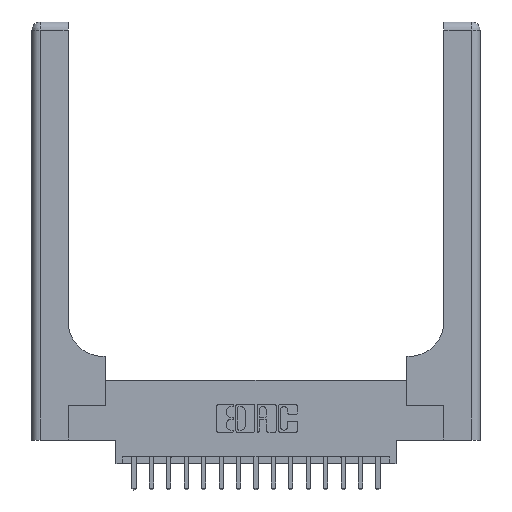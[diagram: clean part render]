
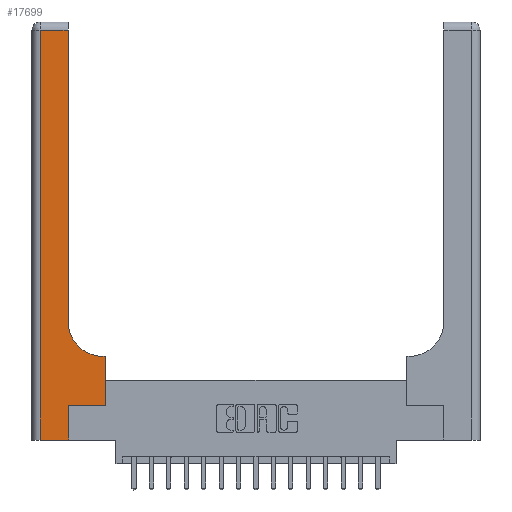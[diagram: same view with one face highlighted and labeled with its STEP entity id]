
A CAD part, top view. The second image highlights one B-rep face of the part: STEP entity #17699.
In plain terms, the highlighted planar face has unit normal (0, 0, 1).
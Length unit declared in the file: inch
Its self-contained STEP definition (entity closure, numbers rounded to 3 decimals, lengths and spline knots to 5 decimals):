
#5 = VERTEX_POINT ( 'NONE', #7284 ) ;
#361 = ORIENTED_EDGE ( 'NONE', *, *, #1503, .T. ) ;
#871 = CARTESIAN_POINT ( 'NONE',  ( 0.265, 0.25, 0.37 ) ) ;
#1188 = ORIENTED_EDGE ( 'NONE', *, *, #7287, .T. ) ;
#1314 = LINE ( 'NONE', #4271, #15556 ) ;
#1371 = CARTESIAN_POINT ( 'NONE',  ( 0.51, 0.6, 0.37 ) ) ;
#1503 = EDGE_CURVE ( 'NONE', #2085, #4782, #2754, .T. ) ;
#1678 = VECTOR ( 'NONE', #9289, 39.37008 ) ;
#1714 = EDGE_CURVE ( 'NONE', #8407, #12423, #7876, .T. ) ;
#2085 = VERTEX_POINT ( 'NONE', #15450 ) ;
#2327 = ORIENTED_EDGE ( 'NONE', *, *, #3861, .T. ) ;
#2394 = CARTESIAN_POINT ( 'NONE',  ( 0.06, 0., 0.37 ) ) ;
#2693 = LINE ( 'NONE', #8613, #10056 ) ;
#2754 = LINE ( 'NONE', #5915, #10117 ) ;
#3510 = DIRECTION ( 'NONE',  ( 1., 0., 0. ) ) ;
#3554 = CARTESIAN_POINT ( 'NONE',  ( 0., 0., 0.37 ) ) ;
#3581 = LINE ( 'NONE', #871, #18537 ) ;
#3772 = CARTESIAN_POINT ( 'NONE',  ( 0.265, 0., 0.37 ) ) ;
#3828 = CARTESIAN_POINT ( 'NONE',  ( 0.06, 2.94, 0.37 ) ) ;
#3861 = EDGE_CURVE ( 'NONE', #13009, #2085, #13807, .T. ) ;
#3913 = CARTESIAN_POINT ( 'NONE',  ( 0.265, 0., 0.37 ) ) ;
#4208 = DIRECTION ( 'NONE',  ( 1., 0., 0. ) ) ;
#4252 = DIRECTION ( 'NONE',  ( 0., 0., -1. ) ) ;
#4258 = CARTESIAN_POINT ( 'NONE',  ( 0.51, 0.85, 0.37 ) ) ;
#4271 = CARTESIAN_POINT ( 'NONE',  ( 0., 2.94, 0.37 ) ) ;
#4648 = ORIENTED_EDGE ( 'NONE', *, *, #17778, .T. ) ;
#4719 = ORIENTED_EDGE ( 'NONE', *, *, #9822, .T. ) ;
#4782 = VERTEX_POINT ( 'NONE', #16737 ) ;
#4795 = VERTEX_POINT ( 'NONE', #15407 ) ;
#5380 = DIRECTION ( 'NONE',  ( 1., 0., 0. ) ) ;
#5852 = DIRECTION ( 'NONE',  ( 0., 1., 0. ) ) ;
#5915 = CARTESIAN_POINT ( 'NONE',  ( 0.26, 3., 0.37 ) ) ;
#6232 = CARTESIAN_POINT ( 'NONE',  ( 0.528, 0.25, 0.37 ) ) ;
#6660 = CARTESIAN_POINT ( 'NONE',  ( 0., 3., 0.37 ) ) ;
#6909 = EDGE_LOOP ( 'NONE', ( #361, #15140, #17762, #6982, #4648, #1188, #4719, #16142, #2327 ) ) ;
#6982 = ORIENTED_EDGE ( 'NONE', *, *, #1714, .T. ) ;
#7284 = CARTESIAN_POINT ( 'NONE',  ( 0.528, 0.25, 0.37 ) ) ;
#7287 = EDGE_CURVE ( 'NONE', #4795, #5, #3581, .T. ) ;
#7313 = LINE ( 'NONE', #3772, #10719 ) ;
#7728 = DIRECTION ( 'NONE',  ( 0., 1., 0. ) ) ;
#7833 = VECTOR ( 'NONE', #7728, 39.37008 ) ;
#7876 = LINE ( 'NONE', #3554, #10815 ) ;
#8159 = DIRECTION ( 'NONE',  ( -1., 0., 0. ) ) ;
#8407 = VERTEX_POINT ( 'NONE', #2394 ) ;
#8613 = CARTESIAN_POINT ( 'NONE',  ( 0.26, 0.6, 0.37 ) ) ;
#8757 = CARTESIAN_POINT ( 'NONE',  ( 0.528, 0.6, 0.37 ) ) ;
#8761 = DIRECTION ( 'NONE',  ( -1., 0., 0. ) ) ;
#9289 = DIRECTION ( 'NONE',  ( 0., -1., 0. ) ) ;
#9431 = VERTEX_POINT ( 'NONE', #3828 ) ;
#9443 = VERTEX_POINT ( 'NONE', #8757 ) ;
#9822 = EDGE_CURVE ( 'NONE', #5, #9443, #12636, .T. ) ;
#10056 = VECTOR ( 'NONE', #18619, 39.37008 ) ;
#10117 = VECTOR ( 'NONE', #5852, 39.37008 ) ;
#10232 = AXIS2_PLACEMENT_3D ( 'NONE', #6660, #16750, #8159 ) ;
#10719 = VECTOR ( 'NONE', #15476, 39.37008 ) ;
#10815 = VECTOR ( 'NONE', #3510, 39.37008 ) ;
#10998 = PLANE ( 'NONE',  #10232 ) ;
#12132 = EDGE_CURVE ( 'NONE', #9431, #8407, #17209, .T. ) ;
#12423 = VERTEX_POINT ( 'NONE', #3913 ) ;
#12598 = AXIS2_PLACEMENT_3D ( 'NONE', #4258, #4252, #4208 ) ;
#12636 = LINE ( 'NONE', #6232, #7833 ) ;
#13009 = VERTEX_POINT ( 'NONE', #1371 ) ;
#13807 = CIRCLE ( 'NONE', #12598, 0.25 ) ;
#15140 = ORIENTED_EDGE ( 'NONE', *, *, #16109, .T. ) ;
#15407 = CARTESIAN_POINT ( 'NONE',  ( 0.265, 0.25, 0.37 ) ) ;
#15450 = CARTESIAN_POINT ( 'NONE',  ( 0.26, 0.85, 0.37 ) ) ;
#15472 = FACE_OUTER_BOUND ( 'NONE', #6909, .T. ) ;
#15476 = DIRECTION ( 'NONE',  ( 0., 1., 0. ) ) ;
#15556 = VECTOR ( 'NONE', #8761, 39.37008 ) ;
#16109 = EDGE_CURVE ( 'NONE', #4782, #9431, #1314, .T. ) ;
#16142 = ORIENTED_EDGE ( 'NONE', *, *, #16703, .T. ) ;
#16466 = CARTESIAN_POINT ( 'NONE',  ( 0.06, 3., 0.37 ) ) ;
#16703 = EDGE_CURVE ( 'NONE', #9443, #13009, #2693, .T. ) ;
#16737 = CARTESIAN_POINT ( 'NONE',  ( 0.26, 2.94, 0.37 ) ) ;
#16750 = DIRECTION ( 'NONE',  ( 0., 0., -1. ) ) ;
#17209 = LINE ( 'NONE', #16466, #1678 ) ;
#17699 = ADVANCED_FACE ( 'NONE', ( #15472 ), #10998, .F. ) ;
#17762 = ORIENTED_EDGE ( 'NONE', *, *, #12132, .T. ) ;
#17778 = EDGE_CURVE ( 'NONE', #12423, #4795, #7313, .T. ) ;
#18537 = VECTOR ( 'NONE', #5380, 39.37008 ) ;
#18619 = DIRECTION ( 'NONE',  ( -1., 0., 0. ) ) ;
